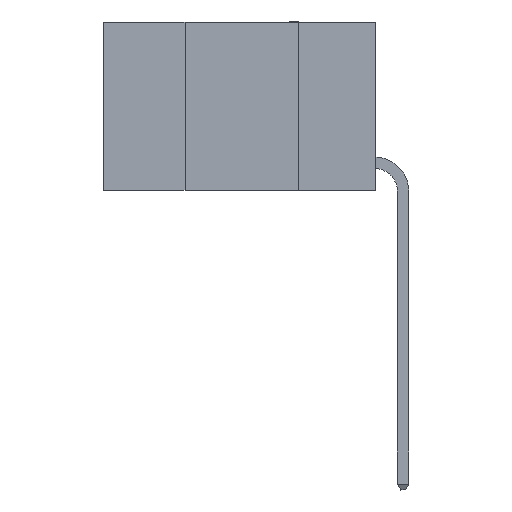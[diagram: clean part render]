
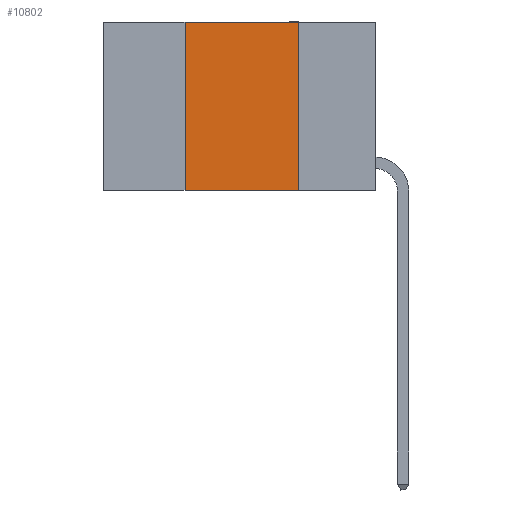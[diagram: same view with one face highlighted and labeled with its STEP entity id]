
A CAD part, left-side view. The second image highlights one B-rep face of the part: STEP entity #10802.
In plain terms, the highlighted planar face has unit normal (-1, 0, 0).
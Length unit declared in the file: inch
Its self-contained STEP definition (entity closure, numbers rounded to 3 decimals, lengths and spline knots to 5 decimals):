
#1267 = DIRECTION ( 'NONE',  ( 0., 0., 1. ) ) ;
#1319 = LINE ( 'NONE', #18417, #22326 ) ;
#1606 = EDGE_CURVE ( 'NONE', #5813, #10543, #6484, .T. ) ;
#1818 = PLANE ( 'NONE',  #13681 ) ;
#3049 = ORIENTED_EDGE ( 'NONE', *, *, #1606, .F. ) ;
#3550 = LINE ( 'NONE', #18835, #8922 ) ;
#3614 = VECTOR ( 'NONE', #19992, 39.37008 ) ;
#4413 = CARTESIAN_POINT ( 'NONE',  ( 0., 0.42, -0.37 ) ) ;
#5456 = FACE_OUTER_BOUND ( 'NONE', #10972, .T. ) ;
#5813 = VERTEX_POINT ( 'NONE', #4413 ) ;
#6207 = CARTESIAN_POINT ( 'NONE',  ( 0., 0.17, 0. ) ) ;
#6222 = VERTEX_POINT ( 'NONE', #9122 ) ;
#6242 = CARTESIAN_POINT ( 'NONE',  ( 0., 0.42, 0. ) ) ;
#6484 = LINE ( 'NONE', #16886, #7653 ) ;
#7653 = VECTOR ( 'NONE', #1267, 39.37008 ) ;
#8015 = LINE ( 'NONE', #6207, #3614 ) ;
#8126 = ORIENTED_EDGE ( 'NONE', *, *, #8776, .T. ) ;
#8167 = VERTEX_POINT ( 'NONE', #12238 ) ;
#8776 = EDGE_CURVE ( 'NONE', #5813, #8167, #1319, .T. ) ;
#8922 = VECTOR ( 'NONE', #17141, 39.37008 ) ;
#9122 = CARTESIAN_POINT ( 'NONE',  ( 0., 0.17, 0. ) ) ;
#9155 = DIRECTION ( 'NONE',  ( 1., 0., 0. ) ) ;
#10220 = EDGE_CURVE ( 'NONE', #10543, #6222, #3550, .T. ) ;
#10543 = VERTEX_POINT ( 'NONE', #6242 ) ;
#10802 = ADVANCED_FACE ( 'NONE', ( #5456 ), #1818, .F. ) ;
#10972 = EDGE_LOOP ( 'NONE', ( #18376, #19943, #3049, #8126 ) ) ;
#12238 = CARTESIAN_POINT ( 'NONE',  ( 0., 0.17, -0.37 ) ) ;
#13478 = EDGE_CURVE ( 'NONE', #6222, #8167, #8015, .T. ) ;
#13681 = AXIS2_PLACEMENT_3D ( 'NONE', #13912, #9155, #19461 ) ;
#13912 = CARTESIAN_POINT ( 'NONE',  ( 0., 0.6, 0. ) ) ;
#16886 = CARTESIAN_POINT ( 'NONE',  ( 0., 0.42, 0. ) ) ;
#17141 = DIRECTION ( 'NONE',  ( 0., -1., 0. ) ) ;
#18376 = ORIENTED_EDGE ( 'NONE', *, *, #13478, .F. ) ;
#18417 = CARTESIAN_POINT ( 'NONE',  ( 0., 0.6, -0.37 ) ) ;
#18835 = CARTESIAN_POINT ( 'NONE',  ( 0., 0.6, 0. ) ) ;
#19461 = DIRECTION ( 'NONE',  ( 0., 0., -1. ) ) ;
#19943 = ORIENTED_EDGE ( 'NONE', *, *, #10220, .F. ) ;
#19992 = DIRECTION ( 'NONE',  ( 0., 0., -1. ) ) ;
#21783 = DIRECTION ( 'NONE',  ( 0., -1., 0. ) ) ;
#22326 = VECTOR ( 'NONE', #21783, 39.37008 ) ;
